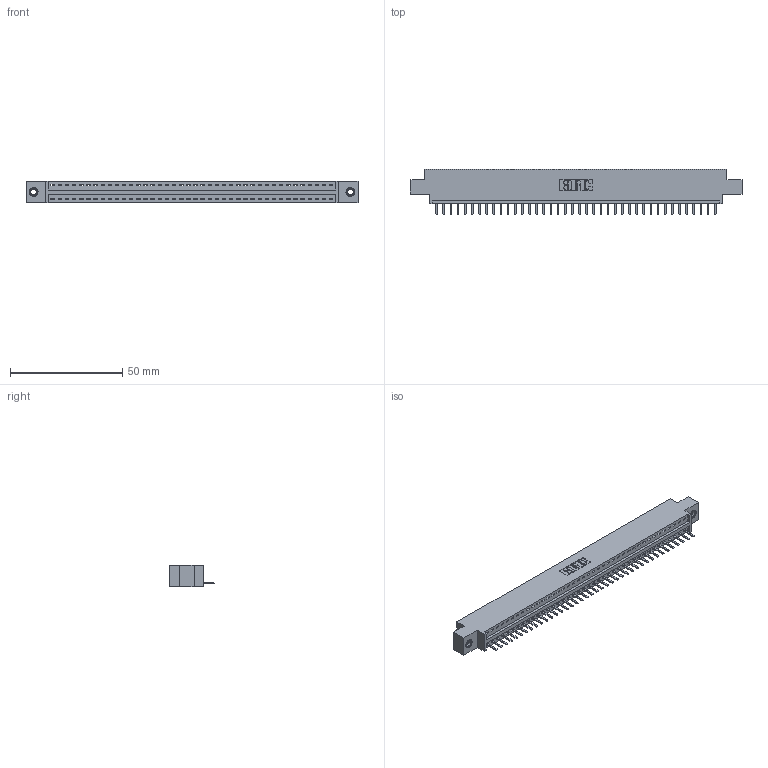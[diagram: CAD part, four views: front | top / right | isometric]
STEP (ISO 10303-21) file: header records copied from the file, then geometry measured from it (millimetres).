
FILE_DESCRIPTION (( 'STEP AP203' ), '1' );
FILE_NAME ('346-040-520-607.STEP', '2022-05-07T08:46:11', ( '' ), ( '' ), 'SwSTEP 2.0', 'SolidWorks 2020', '' );
FILE_SCHEMA (( 'CONFIG_CONTROL_DESIGN' ));
Length unit declared in the file: inch
Products named in the file (4): 345-292-001_345-293-120; 345-250-001_345-250-005-103; 346 Part_0.170 Offset - 0.156 Dia-TI; 346-040-520-607
Assembly tree (43 placements, depth 2):
  346-040-520-607
    346 Part_0.170 Offset - 0.156 Dia-TI
    345-292-001_345-293-120  x40
    345-250-001_345-250-005-103  x2
Bounding box: 147.57 x 20.02 x 9.4 mm (x, y, z)
Volume: 13829.1 mm3; surface area: 17073.9 mm2
Topology: 43 solids, 43 shells, 2666 faces, 7837 edges, 5110 vertices
Faces by surface type: plane 1792, cylinder 858, cone 12, torus 4
Entity records: 26526 total; most frequent: CARTESIAN_POINT 4543, ORIENTED_EDGE 4498, DIRECTION 4023, EDGE_CURVE 2249, LINE 1933, VECTOR 1933, VERTEX_POINT 1492, AXIS2_PLACEMENT_3D 1045
